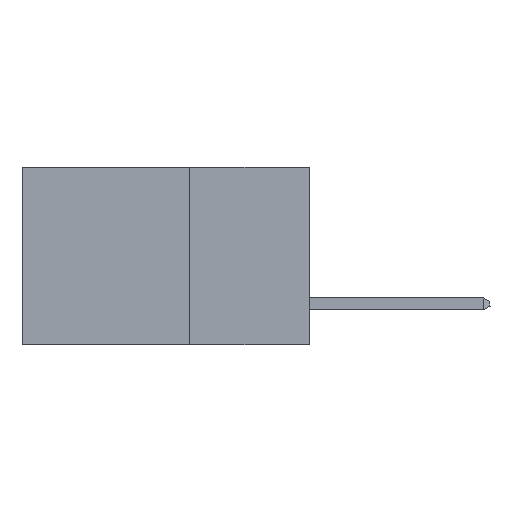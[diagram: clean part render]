
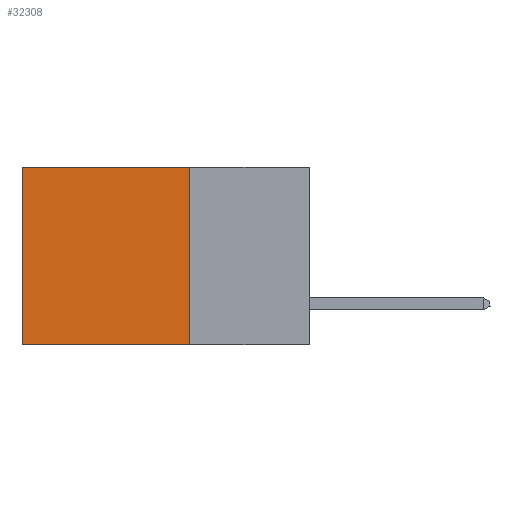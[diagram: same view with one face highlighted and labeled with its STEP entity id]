
A CAD part, left-side view. The second image highlights one B-rep face of the part: STEP entity #32308.
In plain terms, the highlighted planar face has unit normal (-1, 0, 0).
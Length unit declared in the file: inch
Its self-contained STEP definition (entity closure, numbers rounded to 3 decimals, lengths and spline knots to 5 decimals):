
#3548 = ORIENTED_EDGE ( 'NONE', *, *, #28595, .T. ) ;
#3797 = VECTOR ( 'NONE', #36545, 39.37008 ) ;
#4549 = CARTESIAN_POINT ( 'NONE',  ( 0.2875, 0.25, -0.37 ) ) ;
#4841 = ORIENTED_EDGE ( 'NONE', *, *, #29194, .T. ) ;
#6245 = AXIS2_PLACEMENT_3D ( 'NONE', #8611, #33635, #26602 ) ;
#6267 = CARTESIAN_POINT ( 'NONE',  ( 0.2875, 0.6, 0. ) ) ;
#8611 = CARTESIAN_POINT ( 'NONE',  ( 0.2875, 0.25, 0. ) ) ;
#8824 = LINE ( 'NONE', #31711, #3797 ) ;
#10724 = EDGE_CURVE ( 'NONE', #32613, #44039, #32222, .T. ) ;
#13015 = VECTOR ( 'NONE', #24156, 39.37008 ) ;
#14798 = CARTESIAN_POINT ( 'NONE',  ( 0.2875, 0.6, 0. ) ) ;
#15372 = VECTOR ( 'NONE', #30438, 39.37008 ) ;
#16577 = CARTESIAN_POINT ( 'NONE',  ( 0.2875, 0.25, 0. ) ) ;
#17624 = ORIENTED_EDGE ( 'NONE', *, *, #10724, .F. ) ;
#17763 = CARTESIAN_POINT ( 'NONE',  ( 0.2875, 0.6, -0.37 ) ) ;
#18063 = DIRECTION ( 'NONE',  ( 0., 0., -1. ) ) ;
#18342 = CARTESIAN_POINT ( 'NONE',  ( 0.2875, 0.25, 0. ) ) ;
#24156 = DIRECTION ( 'NONE',  ( 0., 1., 0. ) ) ;
#25115 = CARTESIAN_POINT ( 'NONE',  ( 0.2875, 0.25, 0. ) ) ;
#26602 = DIRECTION ( 'NONE',  ( 0., 0., -1. ) ) ;
#26752 = PLANE ( 'NONE',  #6245 ) ;
#28595 = EDGE_CURVE ( 'NONE', #32613, #35058, #32636, .T. ) ;
#29194 = EDGE_CURVE ( 'NONE', #35058, #42901, #29248, .T. ) ;
#29248 = LINE ( 'NONE', #14798, #37665 ) ;
#30438 = DIRECTION ( 'NONE',  ( 0., 0., -1. ) ) ;
#31711 = CARTESIAN_POINT ( 'NONE',  ( 0.2875, 0.25, -0.37 ) ) ;
#32181 = EDGE_CURVE ( 'NONE', #44039, #42901, #8824, .T. ) ;
#32222 = LINE ( 'NONE', #18342, #15372 ) ;
#32308 = ADVANCED_FACE ( 'NONE', ( #44693 ), #26752, .F. ) ;
#32613 = VERTEX_POINT ( 'NONE', #25115 ) ;
#32636 = LINE ( 'NONE', #16577, #13015 ) ;
#33635 = DIRECTION ( 'NONE',  ( 1., 0., 0. ) ) ;
#35058 = VERTEX_POINT ( 'NONE', #6267 ) ;
#36545 = DIRECTION ( 'NONE',  ( 0., 1., 0. ) ) ;
#37665 = VECTOR ( 'NONE', #18063, 39.37008 ) ;
#38072 = ORIENTED_EDGE ( 'NONE', *, *, #32181, .F. ) ;
#42901 = VERTEX_POINT ( 'NONE', #17763 ) ;
#44039 = VERTEX_POINT ( 'NONE', #4549 ) ;
#44693 = FACE_OUTER_BOUND ( 'NONE', #45054, .T. ) ;
#45054 = EDGE_LOOP ( 'NONE', ( #4841, #38072, #17624, #3548 ) ) ;
